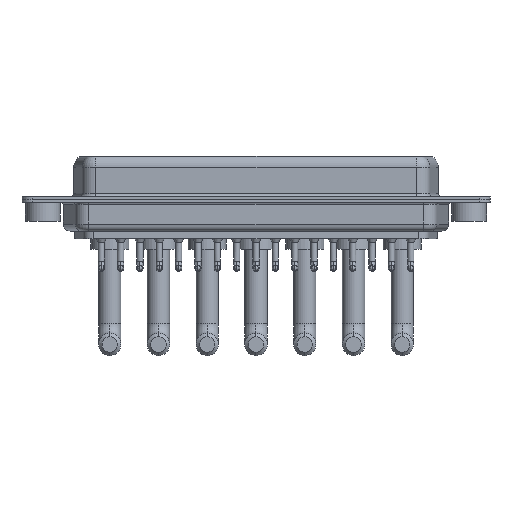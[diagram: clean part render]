
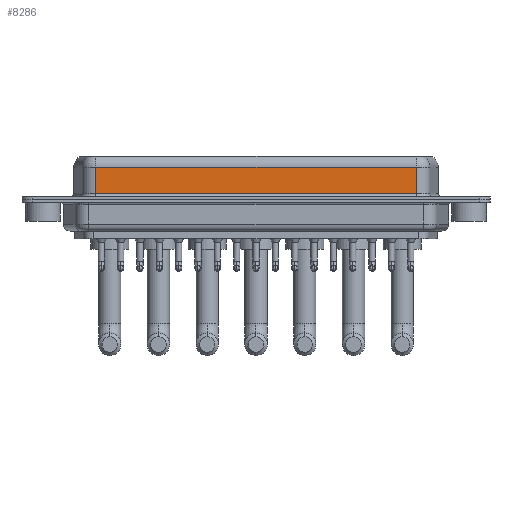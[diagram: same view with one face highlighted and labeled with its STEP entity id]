
A CAD part, front view. The second image highlights one B-rep face of the part: STEP entity #8286.
In plain terms, the highlighted planar face has unit normal (0, -1, 0).
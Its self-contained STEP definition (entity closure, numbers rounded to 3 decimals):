
#355 = CARTESIAN_POINT ( 'NONE',  ( 7.59, -5.375, 4.65 ) ) ;
#2291 = ORIENTED_EDGE ( 'NONE', *, *, #10509, .T. ) ;
#2351 = CARTESIAN_POINT ( 'NONE',  ( 53.41, -5.375, 0.9 ) ) ;
#2884 = DIRECTION ( 'NONE',  ( 0., 0., 1. ) ) ;
#3004 = DIRECTION ( 'NONE',  ( 0., 0., -1. ) ) ;
#3969 = DIRECTION ( 'NONE',  ( 0., 1., 0. ) ) ;
#4147 = VERTEX_POINT ( 'NONE', #355 ) ;
#4621 = CARTESIAN_POINT ( 'NONE',  ( 7.59, -5.375, 6.4 ) ) ;
#4683 = DIRECTION ( 'NONE',  ( -1., 0., 0. ) ) ;
#4949 = CARTESIAN_POINT ( 'NONE',  ( 53.41, -5.375, 4.65 ) ) ;
#5403 = LINE ( 'NONE', #5508, #9924 ) ;
#5508 = CARTESIAN_POINT ( 'NONE',  ( 53.41, -5.375, 6.4 ) ) ;
#6267 = AXIS2_PLACEMENT_3D ( 'NONE', #20643, #3969, #2884 ) ;
#6292 = LINE ( 'NONE', #12693, #7375 ) ;
#6842 = ORIENTED_EDGE ( 'NONE', *, *, #6975, .T. ) ;
#6975 = EDGE_CURVE ( 'NONE', #9651, #4147, #9501, .T. ) ;
#7367 = VERTEX_POINT ( 'NONE', #14688 ) ;
#7375 = VECTOR ( 'NONE', #19428, 1000. ) ;
#8286 = ADVANCED_FACE ( 'NONE', ( #10703 ), #14096, .F. ) ;
#9501 = LINE ( 'NONE', #19320, #16156 ) ;
#9651 = VERTEX_POINT ( 'NONE', #4949 ) ;
#9924 = VECTOR ( 'NONE', #13813, 1000. ) ;
#10509 = EDGE_CURVE ( 'NONE', #7367, #18256, #6292, .T. ) ;
#10703 = FACE_OUTER_BOUND ( 'NONE', #10993, .T. ) ;
#10993 = EDGE_LOOP ( 'NONE', ( #14362, #6842, #19072, #2291 ) ) ;
#12693 = CARTESIAN_POINT ( 'NONE',  ( 53.41, -5.375, 0.9 ) ) ;
#13647 = EDGE_CURVE ( 'NONE', #4147, #7367, #16149, .T. ) ;
#13813 = DIRECTION ( 'NONE',  ( 0., 0., -1. ) ) ;
#14096 = PLANE ( 'NONE',  #6267 ) ;
#14362 = ORIENTED_EDGE ( 'NONE', *, *, #16294, .F. ) ;
#14688 = CARTESIAN_POINT ( 'NONE',  ( 7.59, -5.375, 0.9 ) ) ;
#16149 = LINE ( 'NONE', #4621, #17298 ) ;
#16156 = VECTOR ( 'NONE', #4683, 1000. ) ;
#16294 = EDGE_CURVE ( 'NONE', #9651, #18256, #5403, .T. ) ;
#17298 = VECTOR ( 'NONE', #3004, 1000. ) ;
#18256 = VERTEX_POINT ( 'NONE', #2351 ) ;
#19072 = ORIENTED_EDGE ( 'NONE', *, *, #13647, .T. ) ;
#19320 = CARTESIAN_POINT ( 'NONE',  ( 53.41, -5.375, 4.65 ) ) ;
#19428 = DIRECTION ( 'NONE',  ( 1., 0., 0. ) ) ;
#20643 = CARTESIAN_POINT ( 'NONE',  ( 53.41, -5.375, 6.4 ) ) ;
